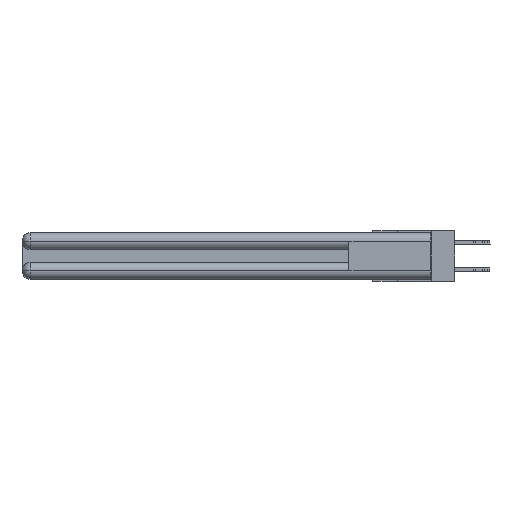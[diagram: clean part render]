
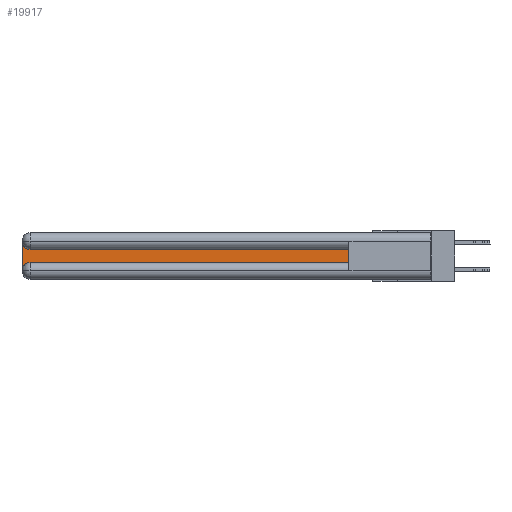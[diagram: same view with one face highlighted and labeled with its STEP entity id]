
A CAD part, left-side view. The second image highlights one B-rep face of the part: STEP entity #19917.
In plain terms, the highlighted planar face has unit normal (-1, 0, 0).
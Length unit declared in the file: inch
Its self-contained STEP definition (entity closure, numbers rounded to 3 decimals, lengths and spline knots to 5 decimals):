
#391 = ORIENTED_EDGE ( 'NONE', *, *, #24080, .T. ) ;
#876 = DIRECTION ( 'NONE',  ( 1., 0., 0. ) ) ;
#4297 = CARTESIAN_POINT ( 'NONE',  ( 0.075, 0.6, -0.2175 ) ) ;
#4339 = CARTESIAN_POINT ( 'NONE',  ( 0.075, 0.6, -0.2175 ) ) ;
#6021 = AXIS2_PLACEMENT_3D ( 'NONE', #7666, #32615, #30305 ) ;
#7035 = LINE ( 'NONE', #26939, #17319 ) ;
#7339 = CARTESIAN_POINT ( 'NONE',  ( 0.075, 3., -0.2175 ) ) ;
#7666 = CARTESIAN_POINT ( 'NONE',  ( 0.075, 3., -0.1225 ) ) ;
#8749 = CARTESIAN_POINT ( 'NONE',  ( 0.075, 2.94, -0.2175 ) ) ;
#10572 = ORIENTED_EDGE ( 'NONE', *, *, #11805, .T. ) ;
#10745 = CARTESIAN_POINT ( 'NONE',  ( 0.075, 2.94, -0.0625 ) ) ;
#10857 = ORIENTED_EDGE ( 'NONE', *, *, #16085, .T. ) ;
#11182 = EDGE_LOOP ( 'NONE', ( #391, #25139, #30082, #10572, #10857, #21949 ) ) ;
#11553 = FACE_OUTER_BOUND ( 'NONE', #11182, .T. ) ;
#11805 = EDGE_CURVE ( 'NONE', #23854, #12584, #19760, .T. ) ;
#11977 = AXIS2_PLACEMENT_3D ( 'NONE', #22149, #24700, #32279 ) ;
#12485 = CARTESIAN_POINT ( 'NONE',  ( 0.075, 0.6, -0.2175 ) ) ;
#12584 = VERTEX_POINT ( 'NONE', #8749 ) ;
#12902 = VECTOR ( 'NONE', #28724, 39.37008 ) ;
#14430 = VERTEX_POINT ( 'NONE', #26486 ) ;
#15117 = DIRECTION ( 'NONE',  ( 0., 1., 0. ) ) ;
#16085 = EDGE_CURVE ( 'NONE', #12584, #19387, #19619, .T. ) ;
#16300 = VECTOR ( 'NONE', #20061, 39.37008 ) ;
#16744 = VERTEX_POINT ( 'NONE', #18225 ) ;
#17065 = DIRECTION ( 'NONE',  ( 0., 0., 1. ) ) ;
#17319 = VECTOR ( 'NONE', #15117, 39.37008 ) ;
#18223 = DIRECTION ( 'NONE',  ( 0., 0., -1. ) ) ;
#18225 = CARTESIAN_POINT ( 'NONE',  ( 0.075, 3., -0.0625 ) ) ;
#19050 = LINE ( 'NONE', #7339, #16300 ) ;
#19214 = EDGE_CURVE ( 'NONE', #28050, #16744, #26258, .T. ) ;
#19387 = VERTEX_POINT ( 'NONE', #12485 ) ;
#19619 = LINE ( 'NONE', #4297, #12902 ) ;
#19754 = EDGE_CURVE ( 'NONE', #19387, #14430, #22224, .T. ) ;
#19760 = CIRCLE ( 'NONE', #11977, 0.06 ) ;
#19855 = EDGE_CURVE ( 'NONE', #16744, #23854, #19050, .T. ) ;
#19917 = ADVANCED_FACE ( 'NONE', ( #11553 ), #32391, .F. ) ;
#20061 = DIRECTION ( 'NONE',  ( 0., 0., -1. ) ) ;
#21949 = ORIENTED_EDGE ( 'NONE', *, *, #19754, .T. ) ;
#22149 = CARTESIAN_POINT ( 'NONE',  ( 0.075, 2.94, -0.2775 ) ) ;
#22224 = LINE ( 'NONE', #4339, #30106 ) ;
#23854 = VERTEX_POINT ( 'NONE', #30945 ) ;
#24080 = EDGE_CURVE ( 'NONE', #14430, #28050, #7035, .T. ) ;
#24700 = DIRECTION ( 'NONE',  ( 1., 0., 0. ) ) ;
#25139 = ORIENTED_EDGE ( 'NONE', *, *, #19214, .T. ) ;
#25212 = CARTESIAN_POINT ( 'NONE',  ( 0.075, 2.94, -0.1225 ) ) ;
#26258 = CIRCLE ( 'NONE', #29263, 0.06 ) ;
#26486 = CARTESIAN_POINT ( 'NONE',  ( 0.075, 0.6, -0.1225 ) ) ;
#26939 = CARTESIAN_POINT ( 'NONE',  ( 0.075, 0.6, -0.1225 ) ) ;
#28050 = VERTEX_POINT ( 'NONE', #25212 ) ;
#28724 = DIRECTION ( 'NONE',  ( 0., -1., 0. ) ) ;
#29263 = AXIS2_PLACEMENT_3D ( 'NONE', #10745, #876, #18223 ) ;
#30082 = ORIENTED_EDGE ( 'NONE', *, *, #19855, .T. ) ;
#30106 = VECTOR ( 'NONE', #17065, 39.37008 ) ;
#30305 = DIRECTION ( 'NONE',  ( 0., 0., -1. ) ) ;
#30945 = CARTESIAN_POINT ( 'NONE',  ( 0.075, 3., -0.2775 ) ) ;
#32279 = DIRECTION ( 'NONE',  ( 0., 0., -1. ) ) ;
#32391 = PLANE ( 'NONE',  #6021 ) ;
#32615 = DIRECTION ( 'NONE',  ( 1., 0., 0. ) ) ;
